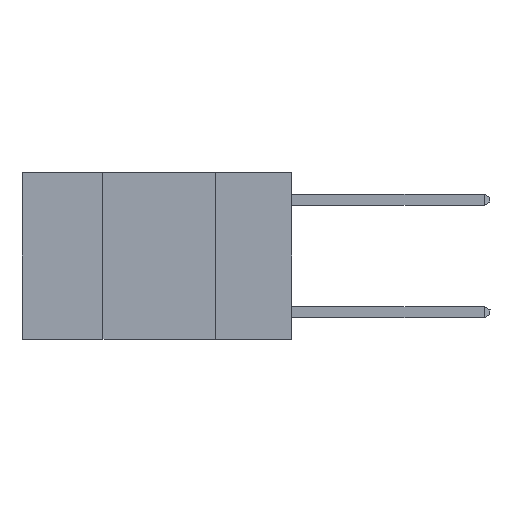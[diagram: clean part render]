
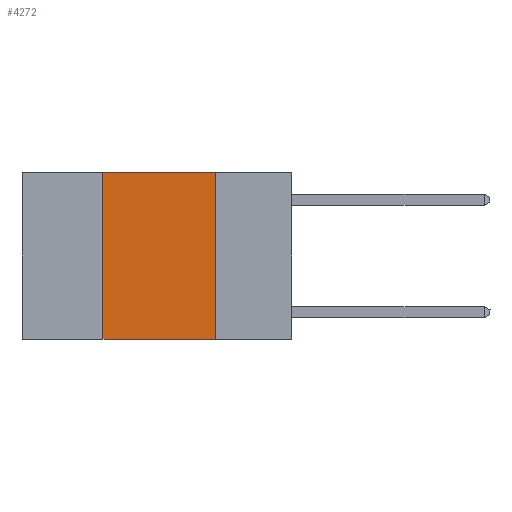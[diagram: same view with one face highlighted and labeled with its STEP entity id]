
A CAD part, left-side view. The second image highlights one B-rep face of the part: STEP entity #4272.
In plain terms, the highlighted planar face has unit normal (-1, 0, 0).
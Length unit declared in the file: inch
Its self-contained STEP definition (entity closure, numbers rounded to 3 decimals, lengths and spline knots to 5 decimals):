
#781 = ORIENTED_EDGE ( 'NONE', *, *, #3941, .F. ) ;
#871 = CARTESIAN_POINT ( 'NONE',  ( 0., 0.42, -0.37 ) ) ;
#1110 = ORIENTED_EDGE ( 'NONE', *, *, #5299, .F. ) ;
#1381 = DIRECTION ( 'NONE',  ( 0., 0., 1. ) ) ;
#1579 = CARTESIAN_POINT ( 'NONE',  ( 0., 0.6, -0.37 ) ) ;
#2105 = CARTESIAN_POINT ( 'NONE',  ( 0., 0.17, 0. ) ) ;
#2851 = EDGE_CURVE ( 'NONE', #19589, #15768, #7200, .T. ) ;
#3411 = ORIENTED_EDGE ( 'NONE', *, *, #8262, .T. ) ;
#3941 = EDGE_CURVE ( 'NONE', #5754, #6386, #16342, .T. ) ;
#4096 = VECTOR ( 'NONE', #1381, 39.37008 ) ;
#4272 = ADVANCED_FACE ( 'NONE', ( #7648 ), #13033, .F. ) ;
#4959 = LINE ( 'NONE', #1579, #8235 ) ;
#5299 = EDGE_CURVE ( 'NONE', #6386, #19589, #11181, .T. ) ;
#5754 = VERTEX_POINT ( 'NONE', #871 ) ;
#6386 = VERTEX_POINT ( 'NONE', #8766 ) ;
#6454 = ORIENTED_EDGE ( 'NONE', *, *, #2851, .F. ) ;
#6496 = DIRECTION ( 'NONE',  ( 0., -1., 0. ) ) ;
#7005 = AXIS2_PLACEMENT_3D ( 'NONE', #17491, #16072, #7044 ) ;
#7026 = DIRECTION ( 'NONE',  ( 0., 0., -1. ) ) ;
#7044 = DIRECTION ( 'NONE',  ( 0., 0., -1. ) ) ;
#7098 = VECTOR ( 'NONE', #10986, 39.37008 ) ;
#7200 = LINE ( 'NONE', #2105, #10353 ) ;
#7648 = FACE_OUTER_BOUND ( 'NONE', #8119, .T. ) ;
#8119 = EDGE_LOOP ( 'NONE', ( #6454, #1110, #781, #3411 ) ) ;
#8235 = VECTOR ( 'NONE', #6496, 39.37008 ) ;
#8262 = EDGE_CURVE ( 'NONE', #5754, #15768, #4959, .T. ) ;
#8766 = CARTESIAN_POINT ( 'NONE',  ( 0., 0.42, 0. ) ) ;
#9394 = CARTESIAN_POINT ( 'NONE',  ( 0., 0.42, 0. ) ) ;
#10353 = VECTOR ( 'NONE', #7026, 39.37008 ) ;
#10986 = DIRECTION ( 'NONE',  ( 0., -1., 0. ) ) ;
#11181 = LINE ( 'NONE', #16882, #7098 ) ;
#11712 = CARTESIAN_POINT ( 'NONE',  ( 0., 0.17, 0. ) ) ;
#13033 = PLANE ( 'NONE',  #7005 ) ;
#15768 = VERTEX_POINT ( 'NONE', #18393 ) ;
#16072 = DIRECTION ( 'NONE',  ( 1., 0., 0. ) ) ;
#16342 = LINE ( 'NONE', #9394, #4096 ) ;
#16882 = CARTESIAN_POINT ( 'NONE',  ( 0., 0.6, 0. ) ) ;
#17491 = CARTESIAN_POINT ( 'NONE',  ( 0., 0.6, 0. ) ) ;
#18393 = CARTESIAN_POINT ( 'NONE',  ( 0., 0.17, -0.37 ) ) ;
#19589 = VERTEX_POINT ( 'NONE', #11712 ) ;
